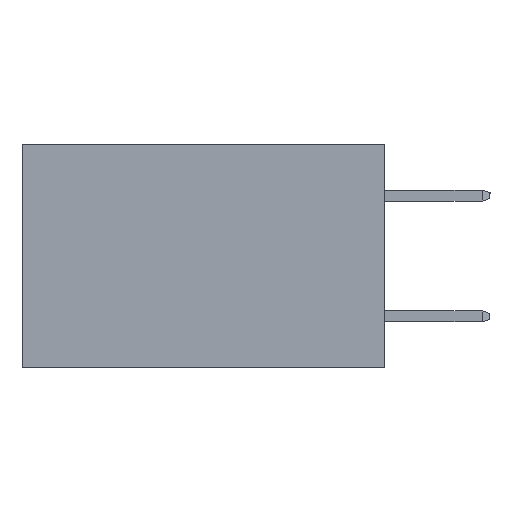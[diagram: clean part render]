
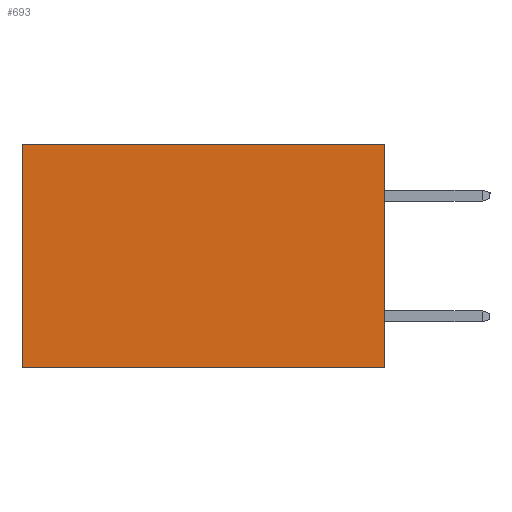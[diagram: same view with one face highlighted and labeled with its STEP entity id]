
A CAD part, left-side view. The second image highlights one B-rep face of the part: STEP entity #693.
In plain terms, the highlighted planar face has unit normal (-1, 0, 0).
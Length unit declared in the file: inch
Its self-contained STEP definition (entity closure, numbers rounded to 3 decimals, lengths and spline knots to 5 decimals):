
#323 = CARTESIAN_POINT ( 'NONE',  ( 0.2615, 0., -0.37 ) ) ;
#537 = ORIENTED_EDGE ( 'NONE', *, *, #4594, .F. ) ;
#693 = ADVANCED_FACE ( 'NONE', ( #1225 ), #3948, .F. ) ;
#729 = VECTOR ( 'NONE', #8612, 39.37008 ) ;
#1063 = CARTESIAN_POINT ( 'NONE',  ( 0.2615, 0., 0. ) ) ;
#1125 = VERTEX_POINT ( 'NONE', #4646 ) ;
#1225 = FACE_OUTER_BOUND ( 'NONE', #4031, .T. ) ;
#1658 = CARTESIAN_POINT ( 'NONE',  ( 0.2615, 0., -0.37 ) ) ;
#1898 = VERTEX_POINT ( 'NONE', #7794 ) ;
#3585 = EDGE_CURVE ( 'NONE', #8021, #9320, #3783, .T. ) ;
#3783 = LINE ( 'NONE', #1063, #4176 ) ;
#3863 = EDGE_CURVE ( 'NONE', #8021, #1898, #9893, .T. ) ;
#3948 = PLANE ( 'NONE',  #10026 ) ;
#3969 = DIRECTION ( 'NONE',  ( 0., 1., 0. ) ) ;
#4031 = EDGE_LOOP ( 'NONE', ( #6729, #537, #9510, #5471 ) ) ;
#4176 = VECTOR ( 'NONE', #3969, 39.37008 ) ;
#4280 = CARTESIAN_POINT ( 'NONE',  ( 0.2615, 0.6, 0. ) ) ;
#4594 = EDGE_CURVE ( 'NONE', #1898, #1125, #6903, .T. ) ;
#4646 = CARTESIAN_POINT ( 'NONE',  ( 0.2615, 0.6, -0.37 ) ) ;
#5027 = DIRECTION ( 'NONE',  ( 1., 0., 0. ) ) ;
#5471 = ORIENTED_EDGE ( 'NONE', *, *, #3585, .T. ) ;
#6046 = LINE ( 'NONE', #10766, #7193 ) ;
#6729 = ORIENTED_EDGE ( 'NONE', *, *, #10647, .T. ) ;
#6903 = LINE ( 'NONE', #10541, #729 ) ;
#7193 = VECTOR ( 'NONE', #9737, 39.37008 ) ;
#7794 = CARTESIAN_POINT ( 'NONE',  ( 0.2615, 0., -0.37 ) ) ;
#8021 = VERTEX_POINT ( 'NONE', #11494 ) ;
#8612 = DIRECTION ( 'NONE',  ( 0., 1., 0. ) ) ;
#9320 = VERTEX_POINT ( 'NONE', #4280 ) ;
#9510 = ORIENTED_EDGE ( 'NONE', *, *, #3863, .F. ) ;
#9737 = DIRECTION ( 'NONE',  ( 0., 0., -1. ) ) ;
#9893 = LINE ( 'NONE', #1658, #11713 ) ;
#10026 = AXIS2_PLACEMENT_3D ( 'NONE', #323, #5027, #10300 ) ;
#10300 = DIRECTION ( 'NONE',  ( 0., 0., -1. ) ) ;
#10541 = CARTESIAN_POINT ( 'NONE',  ( 0.2615, 0., -0.37 ) ) ;
#10647 = EDGE_CURVE ( 'NONE', #9320, #1125, #6046, .T. ) ;
#10766 = CARTESIAN_POINT ( 'NONE',  ( 0.2615, 0.6, -0.37 ) ) ;
#11494 = CARTESIAN_POINT ( 'NONE',  ( 0.2615, 0., 0. ) ) ;
#11713 = VECTOR ( 'NONE', #11817, 39.37008 ) ;
#11817 = DIRECTION ( 'NONE',  ( 0., 0., -1. ) ) ;
